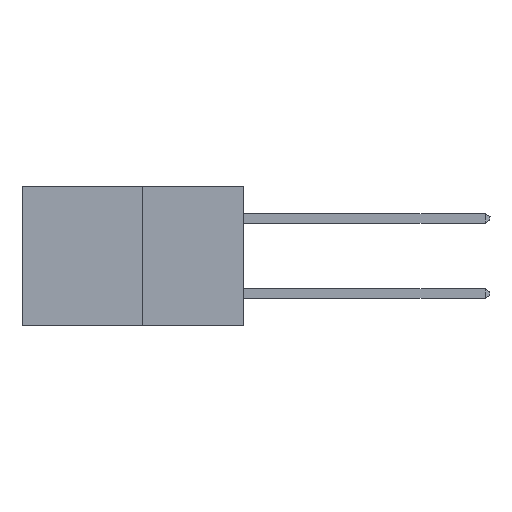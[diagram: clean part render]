
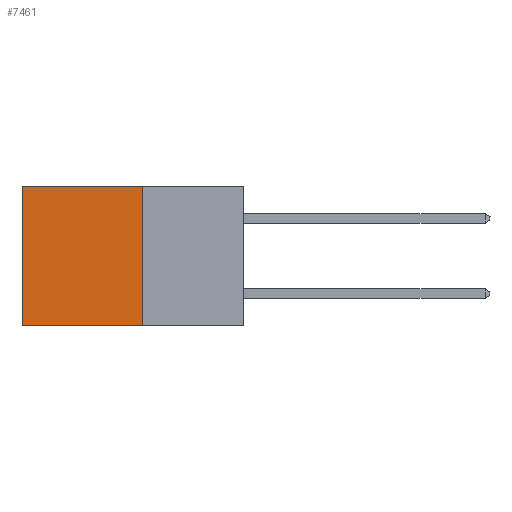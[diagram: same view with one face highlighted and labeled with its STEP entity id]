
A CAD part, left-side view. The second image highlights one B-rep face of the part: STEP entity #7461.
In plain terms, the highlighted planar face has unit normal (-1, 0, 0).
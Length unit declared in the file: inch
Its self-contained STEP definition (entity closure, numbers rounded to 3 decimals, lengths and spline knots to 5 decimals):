
#47 = VECTOR ( 'NONE', #13962, 39.37008 ) ;
#789 = VERTEX_POINT ( 'NONE', #11453 ) ;
#889 = ORIENTED_EDGE ( 'NONE', *, *, #8017, .T. ) ;
#1064 = ORIENTED_EDGE ( 'NONE', *, *, #9892, .T. ) ;
#1623 = CARTESIAN_POINT ( 'NONE',  ( 0.277, 0.27, -0.37 ) ) ;
#1986 = EDGE_CURVE ( 'NONE', #14718, #789, #12480, .T. ) ;
#2050 = LINE ( 'NONE', #6357, #4381 ) ;
#3366 = CARTESIAN_POINT ( 'NONE',  ( 0.277, 0.27, 0. ) ) ;
#3472 = EDGE_LOOP ( 'NONE', ( #1064, #12231, #6688, #889 ) ) ;
#3725 = EDGE_CURVE ( 'NONE', #789, #12889, #13879, .T. ) ;
#4381 = VECTOR ( 'NONE', #6678, 39.37008 ) ;
#4560 = VECTOR ( 'NONE', #11162, 39.37008 ) ;
#4904 = VERTEX_POINT ( 'NONE', #13856 ) ;
#5102 = CARTESIAN_POINT ( 'NONE',  ( 0.277, 0.59, -0.37 ) ) ;
#6357 = CARTESIAN_POINT ( 'NONE',  ( 0.277, 0.27, 0. ) ) ;
#6678 = DIRECTION ( 'NONE',  ( 0., 1., 0. ) ) ;
#6688 = ORIENTED_EDGE ( 'NONE', *, *, #1986, .F. ) ;
#7461 = ADVANCED_FACE ( 'NONE', ( #14567 ), #10822, .F. ) ;
#8017 = EDGE_CURVE ( 'NONE', #14718, #4904, #2050, .T. ) ;
#8831 = AXIS2_PLACEMENT_3D ( 'NONE', #11975, #10491, #10125 ) ;
#9892 = EDGE_CURVE ( 'NONE', #4904, #12889, #13850, .T. ) ;
#10053 = VECTOR ( 'NONE', #12248, 39.37008 ) ;
#10125 = DIRECTION ( 'NONE',  ( 0., 0., -1. ) ) ;
#10491 = DIRECTION ( 'NONE',  ( 1., 0., 0. ) ) ;
#10822 = PLANE ( 'NONE',  #8831 ) ;
#11162 = DIRECTION ( 'NONE',  ( 0., 0., -1. ) ) ;
#11453 = CARTESIAN_POINT ( 'NONE',  ( 0.277, 0.27, -0.37 ) ) ;
#11975 = CARTESIAN_POINT ( 'NONE',  ( 0.277, 0.27, -0.37 ) ) ;
#12231 = ORIENTED_EDGE ( 'NONE', *, *, #3725, .F. ) ;
#12248 = DIRECTION ( 'NONE',  ( 0., 1., 0. ) ) ;
#12480 = LINE ( 'NONE', #1623, #47 ) ;
#12566 = CARTESIAN_POINT ( 'NONE',  ( 0.277, 0.27, -0.37 ) ) ;
#12889 = VERTEX_POINT ( 'NONE', #5102 ) ;
#13419 = CARTESIAN_POINT ( 'NONE',  ( 0.277, 0.59, -0.37 ) ) ;
#13850 = LINE ( 'NONE', #13419, #4560 ) ;
#13856 = CARTESIAN_POINT ( 'NONE',  ( 0.277, 0.59, 0. ) ) ;
#13879 = LINE ( 'NONE', #12566, #10053 ) ;
#13962 = DIRECTION ( 'NONE',  ( 0., 0., -1. ) ) ;
#14567 = FACE_OUTER_BOUND ( 'NONE', #3472, .T. ) ;
#14718 = VERTEX_POINT ( 'NONE', #3366 ) ;
